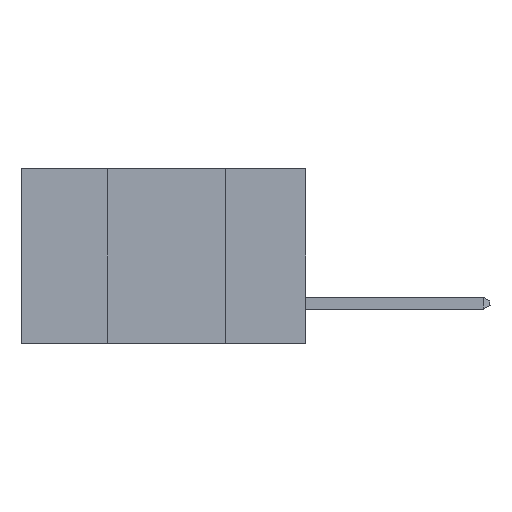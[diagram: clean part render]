
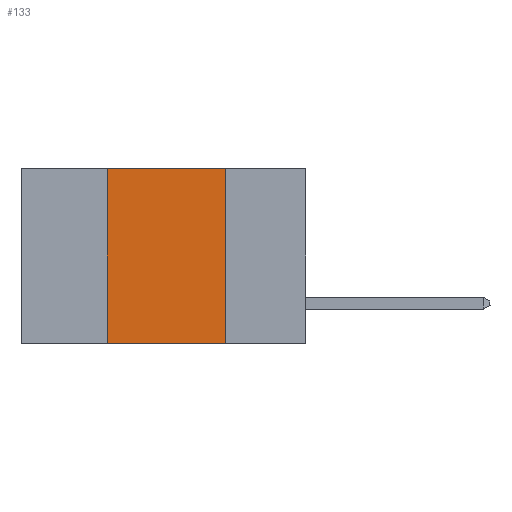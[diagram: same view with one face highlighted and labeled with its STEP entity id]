
A CAD part, left-side view. The second image highlights one B-rep face of the part: STEP entity #133.
In plain terms, the highlighted planar face has unit normal (-1, 0, 0).
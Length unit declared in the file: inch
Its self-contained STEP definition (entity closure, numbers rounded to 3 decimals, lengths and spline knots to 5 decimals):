
#133 = ADVANCED_FACE ( 'NONE', ( #11307 ), #8325, .F. ) ;
#307 = LINE ( 'NONE', #11678, #9205 ) ;
#491 = LINE ( 'NONE', #3968, #5680 ) ;
#1709 = VERTEX_POINT ( 'NONE', #7370 ) ;
#1967 = ORIENTED_EDGE ( 'NONE', *, *, #5505, .T. ) ;
#2020 = EDGE_CURVE ( 'NONE', #8243, #8766, #2785, .T. ) ;
#2245 = CARTESIAN_POINT ( 'NONE',  ( 0., 0.42, 0. ) ) ;
#2693 = CARTESIAN_POINT ( 'NONE',  ( 0., 0.17, 0. ) ) ;
#2785 = LINE ( 'NONE', #11788, #8132 ) ;
#3968 = CARTESIAN_POINT ( 'NONE',  ( 0., 0.17, 0. ) ) ;
#4474 = AXIS2_PLACEMENT_3D ( 'NONE', #5462, #5382, #7279 ) ;
#4500 = VECTOR ( 'NONE', #9491, 39.37008 ) ;
#5382 = DIRECTION ( 'NONE',  ( 1., 0., 0. ) ) ;
#5462 = CARTESIAN_POINT ( 'NONE',  ( 0., 0.6, 0. ) ) ;
#5505 = EDGE_CURVE ( 'NONE', #8243, #1709, #8937, .T. ) ;
#5572 = CARTESIAN_POINT ( 'NONE',  ( 0., 0.6, -0.37 ) ) ;
#5680 = VECTOR ( 'NONE', #9694, 39.37008 ) ;
#6207 = DIRECTION ( 'NONE',  ( 0., 0., 1. ) ) ;
#7033 = CARTESIAN_POINT ( 'NONE',  ( 0., 0.42, -0.37 ) ) ;
#7279 = DIRECTION ( 'NONE',  ( 0., 0., -1. ) ) ;
#7370 = CARTESIAN_POINT ( 'NONE',  ( 0., 0.17, -0.37 ) ) ;
#8132 = VECTOR ( 'NONE', #6207, 39.37008 ) ;
#8243 = VERTEX_POINT ( 'NONE', #7033 ) ;
#8325 = PLANE ( 'NONE',  #4474 ) ;
#8766 = VERTEX_POINT ( 'NONE', #2245 ) ;
#8917 = ORIENTED_EDGE ( 'NONE', *, *, #10102, .F. ) ;
#8921 = DIRECTION ( 'NONE',  ( 0., -1., 0. ) ) ;
#8937 = LINE ( 'NONE', #5572, #4500 ) ;
#9036 = EDGE_CURVE ( 'NONE', #9564, #1709, #491, .T. ) ;
#9205 = VECTOR ( 'NONE', #8921, 39.37008 ) ;
#9491 = DIRECTION ( 'NONE',  ( 0., -1., 0. ) ) ;
#9564 = VERTEX_POINT ( 'NONE', #2693 ) ;
#9694 = DIRECTION ( 'NONE',  ( 0., 0., -1. ) ) ;
#10102 = EDGE_CURVE ( 'NONE', #8766, #9564, #307, .T. ) ;
#11026 = EDGE_LOOP ( 'NONE', ( #11745, #8917, #11329, #1967 ) ) ;
#11307 = FACE_OUTER_BOUND ( 'NONE', #11026, .T. ) ;
#11329 = ORIENTED_EDGE ( 'NONE', *, *, #2020, .F. ) ;
#11678 = CARTESIAN_POINT ( 'NONE',  ( 0., 0.6, 0. ) ) ;
#11745 = ORIENTED_EDGE ( 'NONE', *, *, #9036, .F. ) ;
#11788 = CARTESIAN_POINT ( 'NONE',  ( 0., 0.42, 0. ) ) ;
